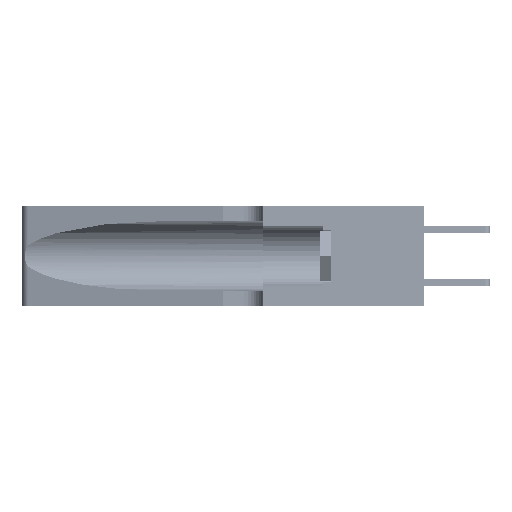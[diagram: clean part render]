
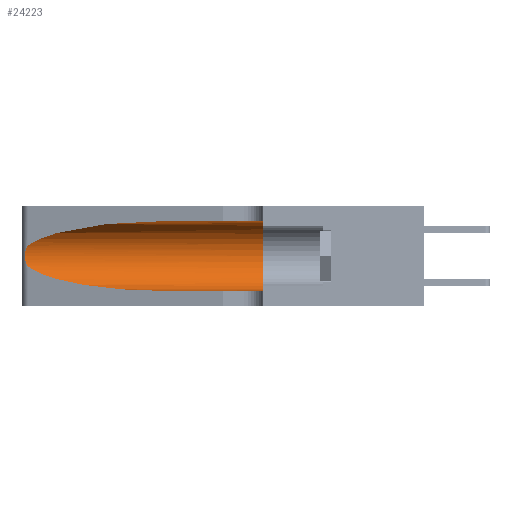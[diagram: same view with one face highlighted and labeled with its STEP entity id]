
A CAD part, left-side view. The second image highlights one B-rep face of the part: STEP entity #24223.
In plain terms, the highlighted cylindrical face has radius 3.308 mm (diameter 6.617 mm), a partial arc.
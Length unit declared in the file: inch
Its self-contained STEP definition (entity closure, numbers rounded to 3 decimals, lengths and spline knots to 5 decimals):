
#63 =( BOUNDED_CURVE ( )  B_SPLINE_CURVE ( 3, ( #20011, #40400, #20358, #12312 ),
 .UNSPECIFIED., .F., .F. ) 
 B_SPLINE_CURVE_WITH_KNOTS ( ( 4, 4 ),
 ( 3.44316, 4.71239 ),
 .UNSPECIFIED. ) 
 CURVE ( )  GEOMETRIC_REPRESENTATION_ITEM ( )  RATIONAL_B_SPLINE_CURVE ( ( 1., 0.87, 0.87, 1. ) ) 
 REPRESENTATION_ITEM ( '' )  );
#1023 = VERTEX_POINT ( 'NONE', #19594 ) ;
#1641 = DIRECTION ( 'NONE',  ( 0., -1., 0. ) ) ;
#3719 = CARTESIAN_POINT ( 'NONE',  ( 0.26017, 1.23833, 0.17102 ) ) ;
#3805 = AXIS2_PLACEMENT_3D ( 'NONE', #15335, #19460, #48423 ) ;
#4319 = ORIENTED_EDGE ( 'NONE', *, *, #26235, .F. ) ;
#4853 = DIRECTION ( 'NONE',  ( 0., 0., 1. ) ) ;
#4933 = VERTEX_POINT ( 'NONE', #36757 ) ;
#5007 = LINE ( 'NONE', #38695, #28189 ) ;
#5155 = VERTEX_POINT ( 'NONE', #14039 ) ;
#6463 = CARTESIAN_POINT ( 'NONE',  ( 0.1305, 0.35, 0.31525 ) ) ;
#7846 = CARTESIAN_POINT ( 'NONE',  ( 0.25487, 1.22718, 0.14631 ) ) ;
#7998 = B_SPLINE_CURVE_WITH_KNOTS ( 'NONE', 3,
 ( #20370, #28351, #32666, #44696, #20022, #36988, #24205, #52979, #3719, #32491, #19857, #12325, #49178, #7846 ),
 .UNSPECIFIED., .F., .F.,
 ( 4, 2, 2, 2, 2, 2, 4 ),
 ( 0., 0.00027, 0.00053, 0.00107, 0.0016, 0.00187, 0.00214 ),
 .UNSPECIFIED. ) ;
#12312 = CARTESIAN_POINT ( 'NONE',  ( 0.1305, 0.72297, 0.05475 ) ) ;
#12325 = CARTESIAN_POINT ( 'NONE',  ( 0.25639, 1.23186, 0.15144 ) ) ;
#13394 = EDGE_CURVE ( 'NONE', #46404, #48009, #7998, .T. ) ;
#14039 = CARTESIAN_POINT ( 'NONE',  ( 0.1305, 0.72297, 0.31525 ) ) ;
#14832 = CARTESIAN_POINT ( 'NONE',  ( 0.25487, 1.22718, 0.22369 ) ) ;
#15335 = CARTESIAN_POINT ( 'NONE',  ( 0.1305, 1.61858, 0.185 ) ) ;
#16730 = ORIENTED_EDGE ( 'NONE', *, *, #13394, .T. ) ;
#17781 = VECTOR ( 'NONE', #22858, 39.37008 ) ;
#19460 = DIRECTION ( 'NONE',  ( 0., -1., 0. ) ) ;
#19594 = CARTESIAN_POINT ( 'NONE',  ( 0.1305, 0.35, 0.05475 ) ) ;
#19857 = CARTESIAN_POINT ( 'NONE',  ( 0.25789, 1.23486, 0.15765 ) ) ;
#20011 = CARTESIAN_POINT ( 'NONE',  ( 0.25487, 1.22718, 0.14631 ) ) ;
#20022 = CARTESIAN_POINT ( 'NONE',  ( 0.25854, 1.2359, 0.20912 ) ) ;
#20358 = CARTESIAN_POINT ( 'NONE',  ( 0.18966, 0.96281, 0.05475 ) ) ;
#20370 = CARTESIAN_POINT ( 'NONE',  ( 0.25487, 1.22718, 0.22369 ) ) ;
#21165 = CARTESIAN_POINT ( 'NONE',  ( 0.1305, 0.35, 0.185 ) ) ;
#21411 = AXIS2_PLACEMENT_3D ( 'NONE', #21165, #28235, #4853 ) ;
#22145 = CIRCLE ( 'NONE', #21411, 0.13025 ) ;
#22858 = DIRECTION ( 'NONE',  ( 0., -1., 0. ) ) ;
#23477 = CARTESIAN_POINT ( 'NONE',  ( 0.18966, 0.96281, 0.31525 ) ) ;
#24205 = CARTESIAN_POINT ( 'NONE',  ( 0.26075, 1.23896, 0.19203 ) ) ;
#24223 = ADVANCED_FACE ( 'NONE', ( #42368 ), #26916, .F. ) ;
#26235 = EDGE_CURVE ( 'NONE', #43009, #1023, #22145, .T. ) ;
#26245 = CARTESIAN_POINT ( 'NONE',  ( 0.25487, 1.22718, 0.22369 ) ) ;
#26916 = CYLINDRICAL_SURFACE ( 'NONE', #3805, 0.13025 ) ;
#27545 = CARTESIAN_POINT ( 'NONE',  ( 0.1305, 1.61858, 0.05475 ) ) ;
#27638 = CARTESIAN_POINT ( 'NONE',  ( 0.2373, 1.15595, 0.28018 ) ) ;
#28189 = VECTOR ( 'NONE', #1641, 39.37008 ) ;
#28235 = DIRECTION ( 'NONE',  ( 0., 1., 0. ) ) ;
#28351 = CARTESIAN_POINT ( 'NONE',  ( 0.25555, 1.22994, 0.2215 ) ) ;
#29114 = ORIENTED_EDGE ( 'NONE', *, *, #39501, .T. ) ;
#30990 = ORIENTED_EDGE ( 'NONE', *, *, #51053, .T. ) ;
#31729 = ORIENTED_EDGE ( 'NONE', *, *, #39646, .T. ) ;
#32491 = CARTESIAN_POINT ( 'NONE',  ( 0.25856, 1.23593, 0.16098 ) ) ;
#32666 = CARTESIAN_POINT ( 'NONE',  ( 0.25639, 1.23184, 0.21858 ) ) ;
#36623 = EDGE_CURVE ( 'NONE', #5155, #43009, #5007, .T. ) ;
#36757 = CARTESIAN_POINT ( 'NONE',  ( 0.1305, 0.72297, 0.05475 ) ) ;
#36988 = CARTESIAN_POINT ( 'NONE',  ( 0.26018, 1.23835, 0.19895 ) ) ;
#38695 = CARTESIAN_POINT ( 'NONE',  ( 0.1305, 1.61858, 0.31525 ) ) ;
#39501 = EDGE_CURVE ( 'NONE', #5155, #46404, #49503, .T. ) ;
#39646 = EDGE_CURVE ( 'NONE', #48009, #4933, #63, .T. ) ;
#40400 = CARTESIAN_POINT ( 'NONE',  ( 0.2373, 1.15595, 0.08982 ) ) ;
#42368 = FACE_OUTER_BOUND ( 'NONE', #48404, .T. ) ;
#43009 = VERTEX_POINT ( 'NONE', #6463 ) ;
#44696 = CARTESIAN_POINT ( 'NONE',  ( 0.25787, 1.23484, 0.2124 ) ) ;
#46404 = VERTEX_POINT ( 'NONE', #26245 ) ;
#48009 = VERTEX_POINT ( 'NONE', #52170 ) ;
#48020 = LINE ( 'NONE', #27545, #17781 ) ;
#48106 = CARTESIAN_POINT ( 'NONE',  ( 0.1305, 0.72297, 0.31525 ) ) ;
#48404 = EDGE_LOOP ( 'NONE', ( #29114, #16730, #31729, #30990, #4319, #50895 ) ) ;
#48423 = DIRECTION ( 'NONE',  ( 0., 0., -1. ) ) ;
#49178 = CARTESIAN_POINT ( 'NONE',  ( 0.25555, 1.22993, 0.14849 ) ) ;
#49503 =( BOUNDED_CURVE ( )  B_SPLINE_CURVE ( 3, ( #48106, #23477, #27638, #14832 ),
 .UNSPECIFIED., .F., .F. ) 
 B_SPLINE_CURVE_WITH_KNOTS ( ( 4, 4 ),
 ( 1.5708, 2.84003 ),
 .UNSPECIFIED. ) 
 CURVE ( )  GEOMETRIC_REPRESENTATION_ITEM ( )  RATIONAL_B_SPLINE_CURVE ( ( 1., 0.87, 0.87, 1. ) ) 
 REPRESENTATION_ITEM ( '' )  );
#50895 = ORIENTED_EDGE ( 'NONE', *, *, #36623, .F. ) ;
#51053 = EDGE_CURVE ( 'NONE', #4933, #1023, #48020, .T. ) ;
#52170 = CARTESIAN_POINT ( 'NONE',  ( 0.25487, 1.22718, 0.14631 ) ) ;
#52979 = CARTESIAN_POINT ( 'NONE',  ( 0.26075, 1.23896, 0.178 ) ) ;
